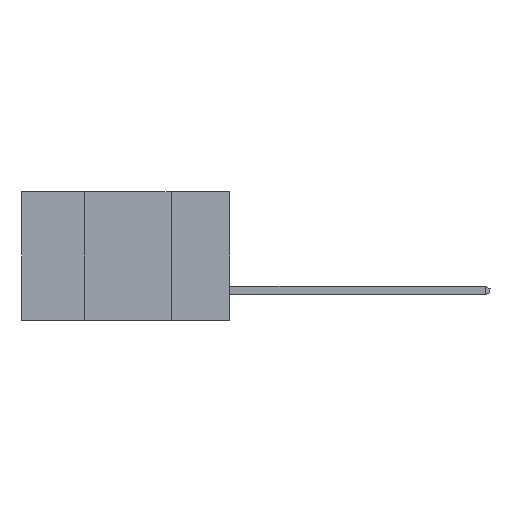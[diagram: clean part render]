
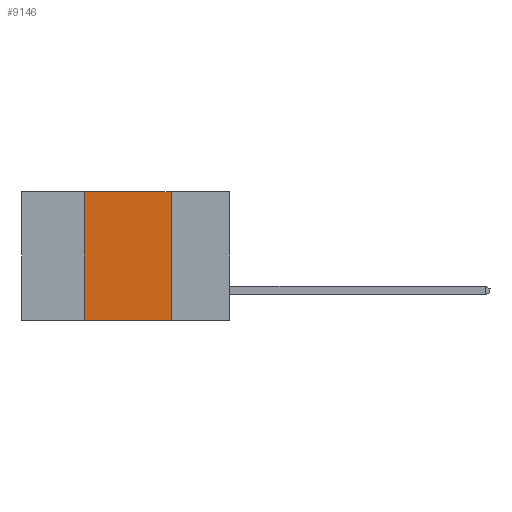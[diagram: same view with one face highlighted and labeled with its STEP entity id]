
A CAD part, left-side view. The second image highlights one B-rep face of the part: STEP entity #9146.
In plain terms, the highlighted planar face has unit normal (-1, 0, 0).
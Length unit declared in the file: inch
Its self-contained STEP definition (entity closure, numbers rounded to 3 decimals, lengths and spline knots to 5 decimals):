
#133 = VECTOR ( 'NONE', #991, 39.37008 ) ;
#212 = EDGE_CURVE ( 'NONE', #13545, #9547, #9400, .T. ) ;
#991 = DIRECTION ( 'NONE',  ( 0., 0., 1. ) ) ;
#1072 = EDGE_CURVE ( 'NONE', #7724, #7878, #11614, .T. ) ;
#1443 = DIRECTION ( 'NONE',  ( 0., -1., 0. ) ) ;
#1906 = CARTESIAN_POINT ( 'NONE',  ( 0., 0.42, -0.37 ) ) ;
#2187 = VECTOR ( 'NONE', #5211, 39.37008 ) ;
#2555 = VECTOR ( 'NONE', #10745, 39.37008 ) ;
#2768 = EDGE_LOOP ( 'NONE', ( #7741, #3859, #9919, #3239 ) ) ;
#2942 = EDGE_CURVE ( 'NONE', #7724, #9547, #4465, .T. ) ;
#3207 = EDGE_CURVE ( 'NONE', #7878, #13545, #6190, .T. ) ;
#3239 = ORIENTED_EDGE ( 'NONE', *, *, #2942, .T. ) ;
#3803 = CARTESIAN_POINT ( 'NONE',  ( 0., 0.6, 0. ) ) ;
#3859 = ORIENTED_EDGE ( 'NONE', *, *, #3207, .F. ) ;
#4465 = LINE ( 'NONE', #5644, #11545 ) ;
#5211 = DIRECTION ( 'NONE',  ( 0., -1., 0. ) ) ;
#5422 = CARTESIAN_POINT ( 'NONE',  ( 0., 0.6, 0. ) ) ;
#5644 = CARTESIAN_POINT ( 'NONE',  ( 0., 0.6, -0.37 ) ) ;
#6113 = PLANE ( 'NONE',  #10333 ) ;
#6190 = LINE ( 'NONE', #5422, #2187 ) ;
#7218 = DIRECTION ( 'NONE',  ( 1., 0., 0. ) ) ;
#7724 = VERTEX_POINT ( 'NONE', #12117 ) ;
#7741 = ORIENTED_EDGE ( 'NONE', *, *, #212, .F. ) ;
#7878 = VERTEX_POINT ( 'NONE', #8248 ) ;
#8248 = CARTESIAN_POINT ( 'NONE',  ( 0., 0.42, 0. ) ) ;
#8284 = CARTESIAN_POINT ( 'NONE',  ( 0., 0.17, -0.37 ) ) ;
#9146 = ADVANCED_FACE ( 'NONE', ( #13592 ), #6113, .F. ) ;
#9400 = LINE ( 'NONE', #8284, #2555 ) ;
#9547 = VERTEX_POINT ( 'NONE', #11741 ) ;
#9919 = ORIENTED_EDGE ( 'NONE', *, *, #1072, .F. ) ;
#10333 = AXIS2_PLACEMENT_3D ( 'NONE', #3803, #7218, #12343 ) ;
#10745 = DIRECTION ( 'NONE',  ( 0., 0., -1. ) ) ;
#11447 = CARTESIAN_POINT ( 'NONE',  ( 0., 0.17, 0. ) ) ;
#11545 = VECTOR ( 'NONE', #1443, 39.37008 ) ;
#11614 = LINE ( 'NONE', #1906, #133 ) ;
#11741 = CARTESIAN_POINT ( 'NONE',  ( 0., 0.17, -0.37 ) ) ;
#12117 = CARTESIAN_POINT ( 'NONE',  ( 0., 0.42, -0.37 ) ) ;
#12343 = DIRECTION ( 'NONE',  ( 0., 0., -1. ) ) ;
#13545 = VERTEX_POINT ( 'NONE', #11447 ) ;
#13592 = FACE_OUTER_BOUND ( 'NONE', #2768, .T. ) ;
